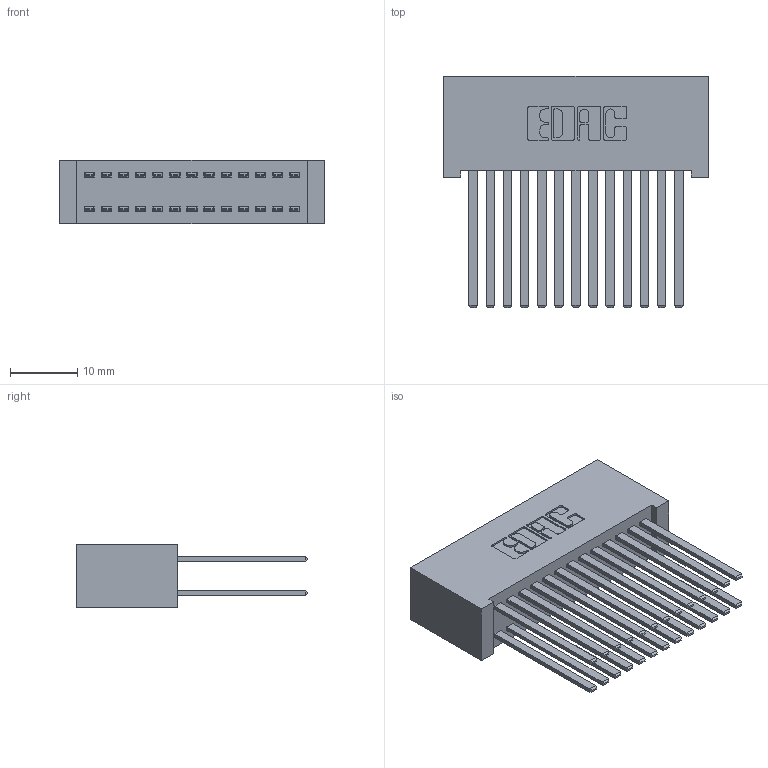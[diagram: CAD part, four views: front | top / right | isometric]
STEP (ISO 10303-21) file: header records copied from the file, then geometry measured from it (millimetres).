
FILE_DESCRIPTION (( 'STEP AP203' ), '1' );
FILE_NAME ('342-026-544-201.STEP', '2018-08-11T04:52:39', ( '' ), ( '' ), 'SwSTEP 2.0', 'SolidWorks 2016', '' );
FILE_SCHEMA (( 'CONFIG_CONTROL_DESIGN' ));
Length unit declared in the file: inch
Products named in the file (3): 342 Part_Lugless; 345-292-001_345-293-144; 342-026-544-201
Assembly tree (27 placements, depth 2):
  342-026-544-201
    342 Part_Lugless
    345-292-001_345-293-144  x26
Bounding box: 39.27 x 34.3 x 9.4 mm (x, y, z)
Volume: 4195 mm3; surface area: 7569.4 mm2
Topology: 27 solids, 27 shells, 1298 faces, 3837 edges, 2522 vertices
Faces by surface type: plane 894, cylinder 404
Entity records: 11521 total; most frequent: CARTESIAN_POINT 1938, ORIENTED_EDGE 1874, DIRECTION 1697, EDGE_CURVE 937, VECTOR 821, LINE 821, VERTEX_POINT 622, AXIS2_PLACEMENT_3D 438
